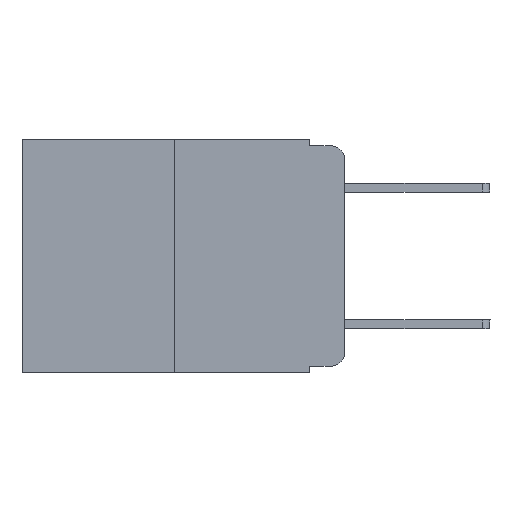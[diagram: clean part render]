
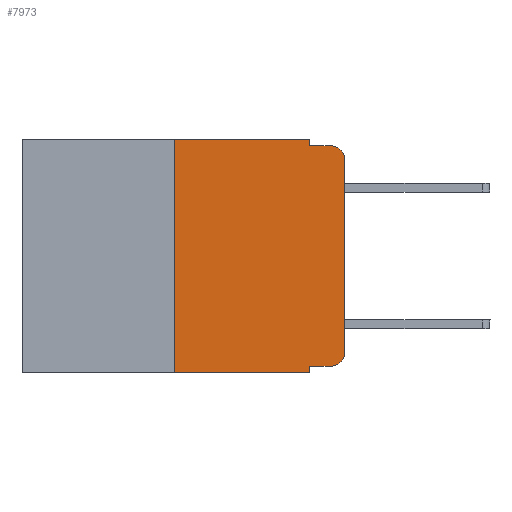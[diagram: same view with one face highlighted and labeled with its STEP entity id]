
A CAD part, left-side view. The second image highlights one B-rep face of the part: STEP entity #7973.
In plain terms, the highlighted planar face has unit normal (-1, 0, 0).
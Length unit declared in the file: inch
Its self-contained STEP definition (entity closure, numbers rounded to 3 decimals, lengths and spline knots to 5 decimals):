
#9 = LINE ( 'NONE', #14172, #8915 ) ;
#77 = EDGE_CURVE ( 'NONE', #12895, #11752, #15255, .T. ) ;
#621 = DIRECTION ( 'NONE',  ( 0., 0., 1. ) ) ;
#834 = LINE ( 'NONE', #20846, #13692 ) ;
#1122 = DIRECTION ( 'NONE',  ( 0., 0., -1. ) ) ;
#1254 = CARTESIAN_POINT ( 'NONE',  ( 0., 0.051, 0. ) ) ;
#1743 = DIRECTION ( 'NONE',  ( 0., -1., 0. ) ) ;
#1748 = DIRECTION ( 'NONE',  ( 0., 0., -1. ) ) ;
#1939 = CARTESIAN_POINT ( 'NONE',  ( 0., 0., 0. ) ) ;
#2042 = VECTOR ( 'NONE', #13939, 39.37008 ) ;
#2159 = VERTEX_POINT ( 'NONE', #20075 ) ;
#2619 = CARTESIAN_POINT ( 'NONE',  ( 0., 0.25, 0. ) ) ;
#2772 = AXIS2_PLACEMENT_3D ( 'NONE', #3200, #2924, #8110 ) ;
#2920 = ORIENTED_EDGE ( 'NONE', *, *, #77, .F. ) ;
#2924 = DIRECTION ( 'NONE',  ( -1., 0., 0. ) ) ;
#3067 = AXIS2_PLACEMENT_3D ( 'NONE', #13242, #4863, #9841 ) ;
#3200 = CARTESIAN_POINT ( 'NONE',  ( 0., 0.02, -0.313 ) ) ;
#3559 = CARTESIAN_POINT ( 'NONE',  ( 0., 0.051, 0. ) ) ;
#3786 = CIRCLE ( 'NONE', #18263, 0.02 ) ;
#3886 = EDGE_LOOP ( 'NONE', ( #7400, #11615, #18947, #10257, #19900, #8383, #10698, #2920, #4858, #20848 ) ) ;
#4019 = DIRECTION ( 'NONE',  ( 0., -1., 0. ) ) ;
#4660 = PLANE ( 'NONE',  #3067 ) ;
#4858 = ORIENTED_EDGE ( 'NONE', *, *, #6924, .T. ) ;
#4863 = DIRECTION ( 'NONE',  ( 1., 0., 0. ) ) ;
#5436 = DIRECTION ( 'NONE',  ( 0., 0., -1. ) ) ;
#5665 = CARTESIAN_POINT ( 'NONE',  ( 0., 0.02, -0.01 ) ) ;
#6583 = VECTOR ( 'NONE', #5436, 39.37008 ) ;
#6924 = EDGE_CURVE ( 'NONE', #12895, #9299, #17276, .T. ) ;
#7312 = CARTESIAN_POINT ( 'NONE',  ( 0., 0.051, -0.01 ) ) ;
#7400 = ORIENTED_EDGE ( 'NONE', *, *, #14730, .T. ) ;
#7803 = LINE ( 'NONE', #10617, #2042 ) ;
#7973 = ADVANCED_FACE ( 'NONE', ( #10101 ), #4660, .F. ) ;
#8110 = DIRECTION ( 'NONE',  ( 0., 0., -1. ) ) ;
#8262 = EDGE_CURVE ( 'NONE', #9299, #13581, #15383, .T. ) ;
#8383 = ORIENTED_EDGE ( 'NONE', *, *, #14910, .F. ) ;
#8547 = CARTESIAN_POINT ( 'NONE',  ( 0., 0.051, -0.343 ) ) ;
#8637 = LINE ( 'NONE', #1939, #21213 ) ;
#8696 = CARTESIAN_POINT ( 'NONE',  ( 0., 0., -0.313 ) ) ;
#8915 = VECTOR ( 'NONE', #621, 39.37008 ) ;
#9140 = CARTESIAN_POINT ( 'NONE',  ( 0., 0.051, -0.01 ) ) ;
#9210 = CARTESIAN_POINT ( 'NONE',  ( 0., 0., -0.03 ) ) ;
#9299 = VERTEX_POINT ( 'NONE', #18295 ) ;
#9382 = EDGE_CURVE ( 'NONE', #17590, #10246, #3786, .T. ) ;
#9841 = DIRECTION ( 'NONE',  ( 0., 0., -1. ) ) ;
#10017 = VECTOR ( 'NONE', #1122, 39.37008 ) ;
#10097 = DIRECTION ( 'NONE',  ( -1., 0., 0. ) ) ;
#10101 = FACE_OUTER_BOUND ( 'NONE', #3886, .T. ) ;
#10214 = EDGE_CURVE ( 'NONE', #2159, #11752, #834, .T. ) ;
#10246 = VERTEX_POINT ( 'NONE', #5665 ) ;
#10257 = ORIENTED_EDGE ( 'NONE', *, *, #10729, .F. ) ;
#10302 = CARTESIAN_POINT ( 'NONE',  ( 0., 0.051, -0.333 ) ) ;
#10617 = CARTESIAN_POINT ( 'NONE',  ( 0., 0.473, 0. ) ) ;
#10698 = ORIENTED_EDGE ( 'NONE', *, *, #10214, .T. ) ;
#10729 = EDGE_CURVE ( 'NONE', #18688, #16345, #19707, .T. ) ;
#11615 = ORIENTED_EDGE ( 'NONE', *, *, #9382, .T. ) ;
#11726 = VECTOR ( 'NONE', #1743, 39.37008 ) ;
#11752 = VERTEX_POINT ( 'NONE', #8547 ) ;
#12895 = VERTEX_POINT ( 'NONE', #10302 ) ;
#13242 = CARTESIAN_POINT ( 'NONE',  ( 0., 0.473, 0. ) ) ;
#13581 = VERTEX_POINT ( 'NONE', #8696 ) ;
#13692 = VECTOR ( 'NONE', #4019, 39.37008 ) ;
#13939 = DIRECTION ( 'NONE',  ( 0., -1., 0. ) ) ;
#14172 = CARTESIAN_POINT ( 'NONE',  ( 0., 0.25, 0. ) ) ;
#14730 = EDGE_CURVE ( 'NONE', #13581, #17590, #8637, .T. ) ;
#14773 = CARTESIAN_POINT ( 'NONE',  ( 0., 0.051, -0.333 ) ) ;
#14910 = EDGE_CURVE ( 'NONE', #2159, #20594, #9, .T. ) ;
#15255 = LINE ( 'NONE', #1254, #10017 ) ;
#15383 = CIRCLE ( 'NONE', #2772, 0.02 ) ;
#15581 = EDGE_CURVE ( 'NONE', #20594, #18688, #7803, .T. ) ;
#16205 = EDGE_CURVE ( 'NONE', #16345, #10246, #17252, .T. ) ;
#16345 = VERTEX_POINT ( 'NONE', #9140 ) ;
#17136 = DIRECTION ( 'NONE',  ( 0., 0., 1. ) ) ;
#17252 = LINE ( 'NONE', #7312, #20623 ) ;
#17276 = LINE ( 'NONE', #14773, #11726 ) ;
#17590 = VERTEX_POINT ( 'NONE', #9210 ) ;
#18263 = AXIS2_PLACEMENT_3D ( 'NONE', #18502, #10097, #1748 ) ;
#18295 = CARTESIAN_POINT ( 'NONE',  ( 0., 0.02, -0.333 ) ) ;
#18502 = CARTESIAN_POINT ( 'NONE',  ( 0., 0.02, -0.03 ) ) ;
#18688 = VERTEX_POINT ( 'NONE', #20354 ) ;
#18907 = DIRECTION ( 'NONE',  ( 0., -1., 0. ) ) ;
#18947 = ORIENTED_EDGE ( 'NONE', *, *, #16205, .F. ) ;
#19707 = LINE ( 'NONE', #3559, #6583 ) ;
#19900 = ORIENTED_EDGE ( 'NONE', *, *, #15581, .F. ) ;
#20075 = CARTESIAN_POINT ( 'NONE',  ( 0., 0.25, -0.343 ) ) ;
#20354 = CARTESIAN_POINT ( 'NONE',  ( 0., 0.051, 0. ) ) ;
#20594 = VERTEX_POINT ( 'NONE', #2619 ) ;
#20623 = VECTOR ( 'NONE', #18907, 39.37008 ) ;
#20846 = CARTESIAN_POINT ( 'NONE',  ( 0., 0.473, -0.343 ) ) ;
#20848 = ORIENTED_EDGE ( 'NONE', *, *, #8262, .T. ) ;
#21213 = VECTOR ( 'NONE', #17136, 39.37008 ) ;
